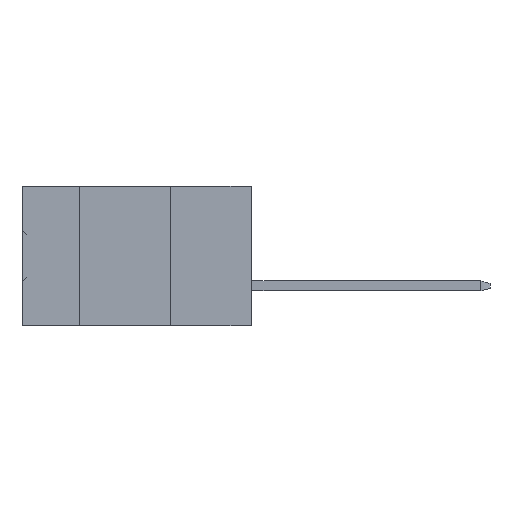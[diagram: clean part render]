
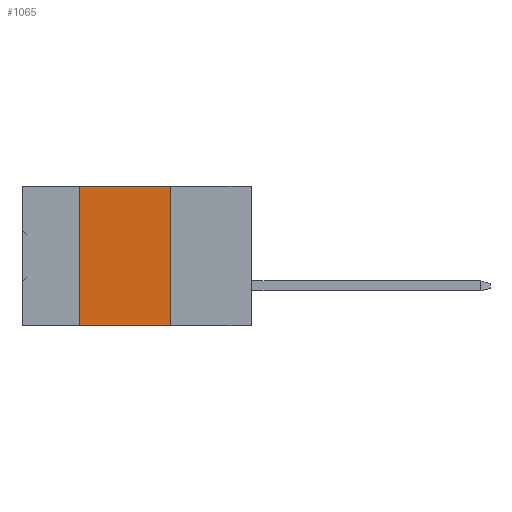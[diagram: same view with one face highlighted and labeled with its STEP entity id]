
A CAD part, left-side view. The second image highlights one B-rep face of the part: STEP entity #1065.
In plain terms, the highlighted planar face has unit normal (-1, 0, 0).
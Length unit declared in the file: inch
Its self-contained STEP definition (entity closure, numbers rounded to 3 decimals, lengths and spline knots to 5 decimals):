
#68 = EDGE_CURVE ( 'NONE', #26521, #427, #4751, .T. ) ;
#73 = DIRECTION ( 'NONE',  ( 1., 0., 0. ) ) ;
#427 = VERTEX_POINT ( 'NONE', #25189 ) ;
#726 = DIRECTION ( 'NONE',  ( 0., 0., -1. ) ) ;
#1065 = ADVANCED_FACE ( 'NONE', ( #10044 ), #30358, .F. ) ;
#4046 = EDGE_CURVE ( 'NONE', #26521, #25703, #4905, .T. ) ;
#4684 = VERTEX_POINT ( 'NONE', #5849 ) ;
#4751 = LINE ( 'NONE', #30363, #13125 ) ;
#4905 = LINE ( 'NONE', #17546, #8538 ) ;
#5849 = CARTESIAN_POINT ( 'NONE',  ( 0., 0.254, 0. ) ) ;
#8538 = VECTOR ( 'NONE', #22887, 39.37008 ) ;
#9726 = VECTOR ( 'NONE', #13007, 39.37008 ) ;
#9843 = VECTOR ( 'NONE', #726, 39.37008 ) ;
#10044 = FACE_OUTER_BOUND ( 'NONE', #26964, .T. ) ;
#11735 = EDGE_CURVE ( 'NONE', #4684, #427, #13867, .T. ) ;
#13007 = DIRECTION ( 'NONE',  ( 0., -1., 0. ) ) ;
#13125 = VECTOR ( 'NONE', #24751, 39.37008 ) ;
#13175 = LINE ( 'NONE', #30474, #9726 ) ;
#13867 = LINE ( 'NONE', #31810, #9843 ) ;
#17495 = CARTESIAN_POINT ( 'NONE',  ( 0., 0.54, -0.437 ) ) ;
#17546 = CARTESIAN_POINT ( 'NONE',  ( 0., 0.54, -0.437 ) ) ;
#19109 = ORIENTED_EDGE ( 'NONE', *, *, #68, .T. ) ;
#19885 = ORIENTED_EDGE ( 'NONE', *, *, #11735, .F. ) ;
#20243 = CARTESIAN_POINT ( 'NONE',  ( 0., 0.72, 0. ) ) ;
#22042 = AXIS2_PLACEMENT_3D ( 'NONE', #20243, #73, #30194 ) ;
#22887 = DIRECTION ( 'NONE',  ( 0., 0., 1. ) ) ;
#23094 = CARTESIAN_POINT ( 'NONE',  ( 0., 0.54, 0. ) ) ;
#24751 = DIRECTION ( 'NONE',  ( 0., -1., 0. ) ) ;
#25189 = CARTESIAN_POINT ( 'NONE',  ( 0., 0.254, -0.437 ) ) ;
#25703 = VERTEX_POINT ( 'NONE', #23094 ) ;
#26366 = ORIENTED_EDGE ( 'NONE', *, *, #29483, .F. ) ;
#26521 = VERTEX_POINT ( 'NONE', #17495 ) ;
#26964 = EDGE_LOOP ( 'NONE', ( #19885, #26366, #29939, #19109 ) ) ;
#29483 = EDGE_CURVE ( 'NONE', #25703, #4684, #13175, .T. ) ;
#29939 = ORIENTED_EDGE ( 'NONE', *, *, #4046, .F. ) ;
#30194 = DIRECTION ( 'NONE',  ( 0., 0., -1. ) ) ;
#30358 = PLANE ( 'NONE',  #22042 ) ;
#30363 = CARTESIAN_POINT ( 'NONE',  ( 0., 0.72, -0.437 ) ) ;
#30474 = CARTESIAN_POINT ( 'NONE',  ( 0., 0.72, 0. ) ) ;
#31810 = CARTESIAN_POINT ( 'NONE',  ( 0., 0.254, -0.437 ) ) ;
